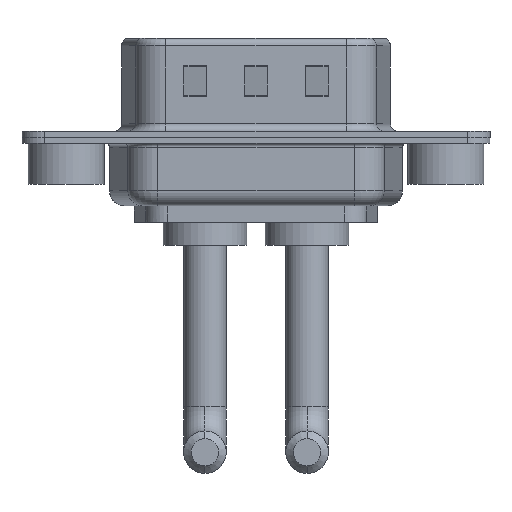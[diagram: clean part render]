
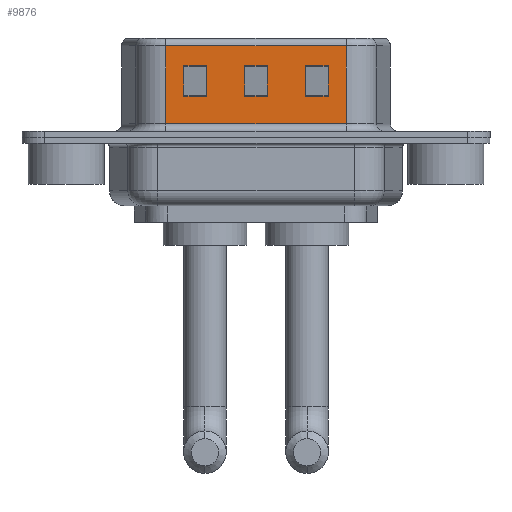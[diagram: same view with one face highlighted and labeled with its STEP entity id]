
A CAD part, front view. The second image highlights one B-rep face of the part: STEP entity #9876.
In plain terms, the highlighted planar face has unit normal (0, -1, 0).
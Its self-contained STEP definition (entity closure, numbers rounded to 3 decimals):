
#13 = EDGE_CURVE ( 'NONE', #12056, #2735, #797, .T. ) ;
#40 = VERTEX_POINT ( 'NONE', #7983 ) ;
#43 = LINE ( 'NONE', #9713, #5908 ) ;
#210 = CARTESIAN_POINT ( 'NONE',  ( 6.549, -4.55, 6.02 ) ) ;
#261 = EDGE_CURVE ( 'NONE', #5814, #11359, #12451, .T. ) ;
#354 = VECTOR ( 'NONE', #11046, 1000. ) ;
#372 = DIRECTION ( 'NONE',  ( 0., 0., -1. ) ) ;
#639 = VERTEX_POINT ( 'NONE', #5534 ) ;
#797 = LINE ( 'NONE', #1009, #6766 ) ;
#804 = CARTESIAN_POINT ( 'NONE',  ( 18.451, -4.55, 2.705 ) ) ;
#815 = CARTESIAN_POINT ( 'NONE',  ( 9.25, -4.55, 2.705 ) ) ;
#1009 = CARTESIAN_POINT ( 'NONE',  ( 15.75, -4.55, 6.52 ) ) ;
#1089 = FACE_BOUND ( 'NONE', #13101, .T. ) ;
#1338 = CARTESIAN_POINT ( 'NONE',  ( 18.451, -4.55, 0.9 ) ) ;
#1707 = VECTOR ( 'NONE', #3497, 1000. ) ;
#1872 = VECTOR ( 'NONE', #3241, 1000. ) ;
#2041 = VERTEX_POINT ( 'NONE', #2537 ) ;
#2072 = CARTESIAN_POINT ( 'NONE',  ( 9.25, -4.55, 6.52 ) ) ;
#2091 = EDGE_CURVE ( 'NONE', #5814, #8572, #9154, .T. ) ;
#2182 = DIRECTION ( 'NONE',  ( -1., 0., 0. ) ) ;
#2273 = LINE ( 'NONE', #11233, #1872 ) ;
#2537 = CARTESIAN_POINT ( 'NONE',  ( 13.25, -4.55, 2.705 ) ) ;
#2541 = LINE ( 'NONE', #6837, #7863 ) ;
#2550 = DIRECTION ( 'NONE',  ( 0., 0., 1. ) ) ;
#2587 = ORIENTED_EDGE ( 'NONE', *, *, #13, .T. ) ;
#2735 = VERTEX_POINT ( 'NONE', #10861 ) ;
#3080 = AXIS2_PLACEMENT_3D ( 'NONE', #12970, #14136, #7707 ) ;
#3218 = LINE ( 'NONE', #804, #5881 ) ;
#3241 = DIRECTION ( 'NONE',  ( 0., 0., 1. ) ) ;
#3255 = LINE ( 'NONE', #2072, #7994 ) ;
#3497 = DIRECTION ( 'NONE',  ( -1., 0., 0. ) ) ;
#3604 = VERTEX_POINT ( 'NONE', #10684 ) ;
#3657 = LINE ( 'NONE', #8075, #7905 ) ;
#3658 = ORIENTED_EDGE ( 'NONE', *, *, #5957, .T. ) ;
#3983 = LINE ( 'NONE', #14106, #6608 ) ;
#4129 = ORIENTED_EDGE ( 'NONE', *, *, #4192, .T. ) ;
#4140 = DIRECTION ( 'NONE',  ( 0., 0., -1. ) ) ;
#4192 = EDGE_CURVE ( 'NONE', #7757, #639, #6064, .T. ) ;
#4210 = CARTESIAN_POINT ( 'NONE',  ( 9.25, -4.55, 4.705 ) ) ;
#4326 = VECTOR ( 'NONE', #14233, 1000. ) ;
#4674 = CARTESIAN_POINT ( 'NONE',  ( 6.549, -4.55, 0.9 ) ) ;
#4944 = VERTEX_POINT ( 'NONE', #12459 ) ;
#5067 = ORIENTED_EDGE ( 'NONE', *, *, #13245, .T. ) ;
#5180 = ORIENTED_EDGE ( 'NONE', *, *, #6883, .T. ) ;
#5264 = DIRECTION ( 'NONE',  ( 0., 0., 1. ) ) ;
#5313 = VECTOR ( 'NONE', #6136, 1000. ) ;
#5368 = DIRECTION ( 'NONE',  ( -1., 0., 0. ) ) ;
#5480 = PLANE ( 'NONE',  #3080 ) ;
#5534 = CARTESIAN_POINT ( 'NONE',  ( 7.75, -4.55, 2.705 ) ) ;
#5779 = ORIENTED_EDGE ( 'NONE', *, *, #8206, .T. ) ;
#5814 = VERTEX_POINT ( 'NONE', #8293 ) ;
#5881 = VECTOR ( 'NONE', #2182, 1000. ) ;
#5908 = VECTOR ( 'NONE', #5368, 1000. ) ;
#5957 = EDGE_CURVE ( 'NONE', #3604, #12397, #7633, .T. ) ;
#6024 = ORIENTED_EDGE ( 'NONE', *, *, #12858, .T. ) ;
#6064 = LINE ( 'NONE', #10483, #5313 ) ;
#6120 = EDGE_CURVE ( 'NONE', #12394, #2041, #2541, .T. ) ;
#6136 = DIRECTION ( 'NONE',  ( -1., 0., 0. ) ) ;
#6370 = VERTEX_POINT ( 'NONE', #11036 ) ;
#6411 = DIRECTION ( 'NONE',  ( 1., 0., 0. ) ) ;
#6601 = CARTESIAN_POINT ( 'NONE',  ( 22.451, -4.55, 4.705 ) ) ;
#6608 = VECTOR ( 'NONE', #4140, 1000. ) ;
#6654 = ORIENTED_EDGE ( 'NONE', *, *, #6120, .T. ) ;
#6731 = DIRECTION ( 'NONE',  ( 1., 0., 0. ) ) ;
#6766 = VECTOR ( 'NONE', #5264, 1000. ) ;
#6813 = ORIENTED_EDGE ( 'NONE', *, *, #9811, .T. ) ;
#6837 = CARTESIAN_POINT ( 'NONE',  ( 13.25, -4.55, 6.52 ) ) ;
#6883 = EDGE_CURVE ( 'NONE', #7523, #11359, #9840, .T. ) ;
#6931 = EDGE_CURVE ( 'NONE', #639, #3604, #2273, .T. ) ;
#6980 = DIRECTION ( 'NONE',  ( 0., 0., -1. ) ) ;
#7478 = VERTEX_POINT ( 'NONE', #12368 ) ;
#7522 = LINE ( 'NONE', #14318, #10565 ) ;
#7523 = VERTEX_POINT ( 'NONE', #4674 ) ;
#7630 = ORIENTED_EDGE ( 'NONE', *, *, #12424, .T. ) ;
#7632 = FACE_OUTER_BOUND ( 'NONE', #12756, .T. ) ;
#7633 = LINE ( 'NONE', #9743, #10665 ) ;
#7707 = DIRECTION ( 'NONE',  ( -1., 0., 0. ) ) ;
#7757 = VERTEX_POINT ( 'NONE', #815 ) ;
#7863 = VECTOR ( 'NONE', #6980, 1000. ) ;
#7905 = VECTOR ( 'NONE', #2550, 1000. ) ;
#7983 = CARTESIAN_POINT ( 'NONE',  ( 11.75, -4.55, 4.705 ) ) ;
#7994 = VECTOR ( 'NONE', #12114, 1000. ) ;
#8075 = CARTESIAN_POINT ( 'NONE',  ( 11.75, -4.55, 6.52 ) ) ;
#8206 = EDGE_CURVE ( 'NONE', #4944, #40, #3657, .T. ) ;
#8293 = CARTESIAN_POINT ( 'NONE',  ( 18.451, -4.55, 6.02 ) ) ;
#8572 = VERTEX_POINT ( 'NONE', #210 ) ;
#9154 = LINE ( 'NONE', #10319, #1707 ) ;
#9156 = ORIENTED_EDGE ( 'NONE', *, *, #261, .F. ) ;
#9163 = CARTESIAN_POINT ( 'NONE',  ( 18.451, -4.55, 6.52 ) ) ;
#9713 = CARTESIAN_POINT ( 'NONE',  ( 22.451, -4.55, 2.705 ) ) ;
#9714 = CARTESIAN_POINT ( 'NONE',  ( 13.25, -4.55, 4.705 ) ) ;
#9743 = CARTESIAN_POINT ( 'NONE',  ( 14.451, -4.55, 4.705 ) ) ;
#9772 = CARTESIAN_POINT ( 'NONE',  ( 6.549, -4.55, 6.52 ) ) ;
#9811 = EDGE_CURVE ( 'NONE', #2041, #4944, #3218, .T. ) ;
#9815 = FACE_BOUND ( 'NONE', #14330, .T. ) ;
#9840 = LINE ( 'NONE', #13355, #11412 ) ;
#9869 = LINE ( 'NONE', #6601, #354 ) ;
#9876 = ADVANCED_FACE ( 'NONE', ( #11870, #9815, #1089, #7632 ), #5480, .F. ) ;
#10065 = LINE ( 'NONE', #9772, #4326 ) ;
#10236 = VECTOR ( 'NONE', #372, 1000. ) ;
#10319 = CARTESIAN_POINT ( 'NONE',  ( 18.451, -4.55, 6.02 ) ) ;
#10483 = CARTESIAN_POINT ( 'NONE',  ( 14.451, -4.55, 2.705 ) ) ;
#10565 = VECTOR ( 'NONE', #6731, 1000. ) ;
#10665 = VECTOR ( 'NONE', #6411, 1000. ) ;
#10684 = CARTESIAN_POINT ( 'NONE',  ( 7.75, -4.55, 4.705 ) ) ;
#10861 = CARTESIAN_POINT ( 'NONE',  ( 15.75, -4.55, 4.705 ) ) ;
#11036 = CARTESIAN_POINT ( 'NONE',  ( 17.25, -4.55, 2.705 ) ) ;
#11046 = DIRECTION ( 'NONE',  ( 1., 0., 0. ) ) ;
#11233 = CARTESIAN_POINT ( 'NONE',  ( 7.75, -4.55, 6.52 ) ) ;
#11244 = EDGE_CURVE ( 'NONE', #6370, #12056, #43, .T. ) ;
#11359 = VERTEX_POINT ( 'NONE', #1338 ) ;
#11412 = VECTOR ( 'NONE', #13489, 1000. ) ;
#11870 = FACE_BOUND ( 'NONE', #12115, .T. ) ;
#11953 = ORIENTED_EDGE ( 'NONE', *, *, #6931, .T. ) ;
#12056 = VERTEX_POINT ( 'NONE', #12135 ) ;
#12114 = DIRECTION ( 'NONE',  ( 0., 0., -1. ) ) ;
#12115 = EDGE_LOOP ( 'NONE', ( #7630, #4129, #11953, #3658 ) ) ;
#12135 = CARTESIAN_POINT ( 'NONE',  ( 15.75, -4.55, 2.705 ) ) ;
#12368 = CARTESIAN_POINT ( 'NONE',  ( 17.25, -4.55, 4.705 ) ) ;
#12381 = EDGE_CURVE ( 'NONE', #7478, #6370, #3983, .T. ) ;
#12394 = VERTEX_POINT ( 'NONE', #9714 ) ;
#12397 = VERTEX_POINT ( 'NONE', #4210 ) ;
#12424 = EDGE_CURVE ( 'NONE', #12397, #7757, #3255, .T. ) ;
#12451 = LINE ( 'NONE', #9163, #10236 ) ;
#12459 = CARTESIAN_POINT ( 'NONE',  ( 11.75, -4.55, 2.705 ) ) ;
#12567 = EDGE_CURVE ( 'NONE', #40, #12394, #7522, .T. ) ;
#12756 = EDGE_LOOP ( 'NONE', ( #9156, #13643, #5067, #5180 ) ) ;
#12858 = EDGE_CURVE ( 'NONE', #2735, #7478, #9869, .T. ) ;
#12970 = CARTESIAN_POINT ( 'NONE',  ( 18.451, -4.55, 6.52 ) ) ;
#13101 = EDGE_LOOP ( 'NONE', ( #13777, #6654, #6813, #5779 ) ) ;
#13157 = ORIENTED_EDGE ( 'NONE', *, *, #12381, .T. ) ;
#13245 = EDGE_CURVE ( 'NONE', #8572, #7523, #10065, .T. ) ;
#13300 = ORIENTED_EDGE ( 'NONE', *, *, #11244, .T. ) ;
#13355 = CARTESIAN_POINT ( 'NONE',  ( 18.451, -4.55, 0.9 ) ) ;
#13489 = DIRECTION ( 'NONE',  ( 1., 0., 0. ) ) ;
#13643 = ORIENTED_EDGE ( 'NONE', *, *, #2091, .T. ) ;
#13777 = ORIENTED_EDGE ( 'NONE', *, *, #12567, .T. ) ;
#14106 = CARTESIAN_POINT ( 'NONE',  ( 17.25, -4.55, 6.52 ) ) ;
#14136 = DIRECTION ( 'NONE',  ( 0., 1., 0. ) ) ;
#14233 = DIRECTION ( 'NONE',  ( 0., 0., -1. ) ) ;
#14318 = CARTESIAN_POINT ( 'NONE',  ( 18.451, -4.55, 4.705 ) ) ;
#14330 = EDGE_LOOP ( 'NONE', ( #13157, #13300, #2587, #6024 ) ) ;
